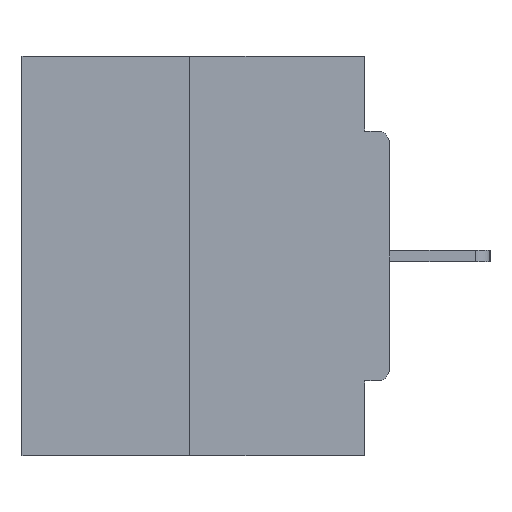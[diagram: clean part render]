
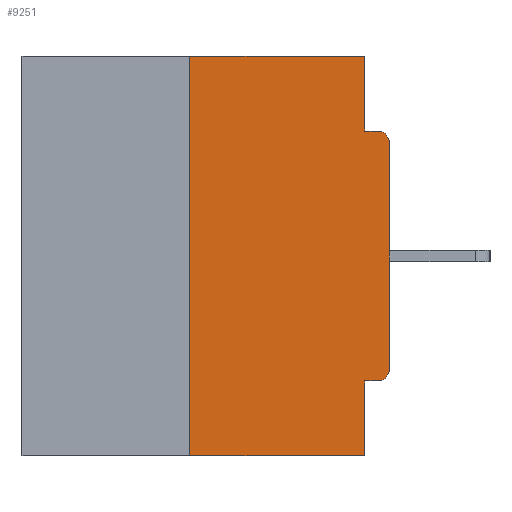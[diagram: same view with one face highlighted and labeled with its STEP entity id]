
A CAD part, left-side view. The second image highlights one B-rep face of the part: STEP entity #9251.
In plain terms, the highlighted planar face has unit normal (-1, 0, 0).
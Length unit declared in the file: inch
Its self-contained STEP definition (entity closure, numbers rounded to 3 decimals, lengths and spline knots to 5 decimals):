
#440 = VERTEX_POINT ( 'NONE', #9638 ) ;
#1334 = CARTESIAN_POINT ( 'NONE',  ( 0., 0.46, 0. ) ) ;
#1359 = DIRECTION ( 'NONE',  ( -1., 0., 0. ) ) ;
#1471 = DIRECTION ( 'NONE',  ( 0., 0., -1. ) ) ;
#1513 = CARTESIAN_POINT ( 'NONE',  ( 0., 0., -0.3915 ) ) ;
#1755 = VECTOR ( 'NONE', #20058, 39.37008 ) ;
#1803 = CARTESIAN_POINT ( 'NONE',  ( 0., 0.031, -0.4065 ) ) ;
#2010 = VERTEX_POINT ( 'NONE', #21526 ) ;
#2315 = LINE ( 'NONE', #20993, #14277 ) ;
#2349 = CARTESIAN_POINT ( 'NONE',  ( 0., 0.46, -0.5 ) ) ;
#2356 = ORIENTED_EDGE ( 'NONE', *, *, #29031, .F. ) ;
#3362 = DIRECTION ( 'NONE',  ( 0., -1., 0. ) ) ;
#3438 = LINE ( 'NONE', #2349, #16137 ) ;
#3883 = VERTEX_POINT ( 'NONE', #31099 ) ;
#3939 = DIRECTION ( 'NONE',  ( 1., 0., 0. ) ) ;
#4921 = DIRECTION ( 'NONE',  ( 0., -1., 0. ) ) ;
#4940 = DIRECTION ( 'NONE',  ( 0., 1., 0. ) ) ;
#5455 = EDGE_CURVE ( 'NONE', #22791, #25155, #29235, .T. ) ;
#6534 = ORIENTED_EDGE ( 'NONE', *, *, #11561, .F. ) ;
#6559 = ORIENTED_EDGE ( 'NONE', *, *, #30650, .F. ) ;
#6981 = LINE ( 'NONE', #16709, #25346 ) ;
#7410 = CARTESIAN_POINT ( 'NONE',  ( 0., 0.031, -0.5 ) ) ;
#7814 = LINE ( 'NONE', #27612, #28419 ) ;
#8474 = ORIENTED_EDGE ( 'NONE', *, *, #28523, .T. ) ;
#9191 = EDGE_LOOP ( 'NONE', ( #6534, #6559, #8474, #9258, #11712, #14458, #14517, #18495, #21817, #2356 ) ) ;
#9251 = ADVANCED_FACE ( 'NONE', ( #13183 ), #28791, .F. ) ;
#9258 = ORIENTED_EDGE ( 'NONE', *, *, #27959, .F. ) ;
#9502 = VECTOR ( 'NONE', #11062, 39.37008 ) ;
#9638 = CARTESIAN_POINT ( 'NONE',  ( 0., 0.031, -0.0935 ) ) ;
#10533 = CARTESIAN_POINT ( 'NONE',  ( 0., 0.031, -0.5 ) ) ;
#11062 = DIRECTION ( 'NONE',  ( 0., 0., 1. ) ) ;
#11561 = EDGE_CURVE ( 'NONE', #2010, #16610, #2315, .T. ) ;
#11712 = ORIENTED_EDGE ( 'NONE', *, *, #5455, .F. ) ;
#12018 = VECTOR ( 'NONE', #25767, 39.37008 ) ;
#12035 = VERTEX_POINT ( 'NONE', #18309 ) ;
#13183 = FACE_OUTER_BOUND ( 'NONE', #9191, .T. ) ;
#13267 = CIRCLE ( 'NONE', #13979, 0.015 ) ;
#13546 = CARTESIAN_POINT ( 'NONE',  ( 0., 0.015, -0.1085 ) ) ;
#13979 = AXIS2_PLACEMENT_3D ( 'NONE', #13546, #30703, #16085 ) ;
#14277 = VECTOR ( 'NONE', #3362, 39.37008 ) ;
#14458 = ORIENTED_EDGE ( 'NONE', *, *, #25045, .T. ) ;
#14517 = ORIENTED_EDGE ( 'NONE', *, *, #26025, .T. ) ;
#15047 = AXIS2_PLACEMENT_3D ( 'NONE', #16602, #1359, #19093 ) ;
#15344 = EDGE_CURVE ( 'NONE', #3883, #22470, #13267, .T. ) ;
#16085 = DIRECTION ( 'NONE',  ( 0., 0., -1. ) ) ;
#16137 = VECTOR ( 'NONE', #4921, 39.37008 ) ;
#16602 = CARTESIAN_POINT ( 'NONE',  ( 0., 0.015, -0.3915 ) ) ;
#16610 = VERTEX_POINT ( 'NONE', #25803 ) ;
#16709 = CARTESIAN_POINT ( 'NONE',  ( 0., 0.031, 0. ) ) ;
#16993 = VECTOR ( 'NONE', #4940, 39.37008 ) ;
#18309 = CARTESIAN_POINT ( 'NONE',  ( 0., 0.25, -0.5 ) ) ;
#18495 = ORIENTED_EDGE ( 'NONE', *, *, #15344, .T. ) ;
#18877 = VERTEX_POINT ( 'NONE', #1513 ) ;
#19093 = DIRECTION ( 'NONE',  ( 0., 0., -1. ) ) ;
#19469 = LINE ( 'NONE', #20737, #12018 ) ;
#20058 = DIRECTION ( 'NONE',  ( 0., 0., -1. ) ) ;
#20737 = CARTESIAN_POINT ( 'NONE',  ( 0., 0.25, 0. ) ) ;
#20982 = CARTESIAN_POINT ( 'NONE',  ( 0., 0., 0. ) ) ;
#20993 = CARTESIAN_POINT ( 'NONE',  ( 0., 0.46, 0. ) ) ;
#21526 = CARTESIAN_POINT ( 'NONE',  ( 0., 0.25, 0. ) ) ;
#21551 = DIRECTION ( 'NONE',  ( 0., 0., -1. ) ) ;
#21817 = ORIENTED_EDGE ( 'NONE', *, *, #28600, .F. ) ;
#22318 = AXIS2_PLACEMENT_3D ( 'NONE', #1334, #3939, #21551 ) ;
#22354 = CARTESIAN_POINT ( 'NONE',  ( 0., 0.015, -0.4065 ) ) ;
#22470 = VERTEX_POINT ( 'NONE', #28447 ) ;
#22750 = LINE ( 'NONE', #20982, #9502 ) ;
#22791 = VERTEX_POINT ( 'NONE', #22354 ) ;
#23703 = CARTESIAN_POINT ( 'NONE',  ( 0., 0., -0.4065 ) ) ;
#25045 = EDGE_CURVE ( 'NONE', #22791, #18877, #30790, .T. ) ;
#25155 = VERTEX_POINT ( 'NONE', #1803 ) ;
#25346 = VECTOR ( 'NONE', #1471, 39.37008 ) ;
#25767 = DIRECTION ( 'NONE',  ( 0., 0., 1. ) ) ;
#25803 = CARTESIAN_POINT ( 'NONE',  ( 0., 0.031, 0. ) ) ;
#26025 = EDGE_CURVE ( 'NONE', #18877, #3883, #22750, .T. ) ;
#27612 = CARTESIAN_POINT ( 'NONE',  ( 0., 0., -0.0935 ) ) ;
#27959 = EDGE_CURVE ( 'NONE', #25155, #28657, #28388, .T. ) ;
#28388 = LINE ( 'NONE', #7410, #1755 ) ;
#28419 = VECTOR ( 'NONE', #30005, 39.37008 ) ;
#28447 = CARTESIAN_POINT ( 'NONE',  ( 0., 0.015, -0.0935 ) ) ;
#28523 = EDGE_CURVE ( 'NONE', #12035, #28657, #3438, .T. ) ;
#28600 = EDGE_CURVE ( 'NONE', #440, #22470, #7814, .T. ) ;
#28657 = VERTEX_POINT ( 'NONE', #10533 ) ;
#28791 = PLANE ( 'NONE',  #22318 ) ;
#29031 = EDGE_CURVE ( 'NONE', #16610, #440, #6981, .T. ) ;
#29235 = LINE ( 'NONE', #23703, #16993 ) ;
#30005 = DIRECTION ( 'NONE',  ( 0., -1., 0. ) ) ;
#30650 = EDGE_CURVE ( 'NONE', #12035, #2010, #19469, .T. ) ;
#30703 = DIRECTION ( 'NONE',  ( -1., 0., 0. ) ) ;
#30790 = CIRCLE ( 'NONE', #15047, 0.015 ) ;
#31099 = CARTESIAN_POINT ( 'NONE',  ( 0., 0., -0.1085 ) ) ;
